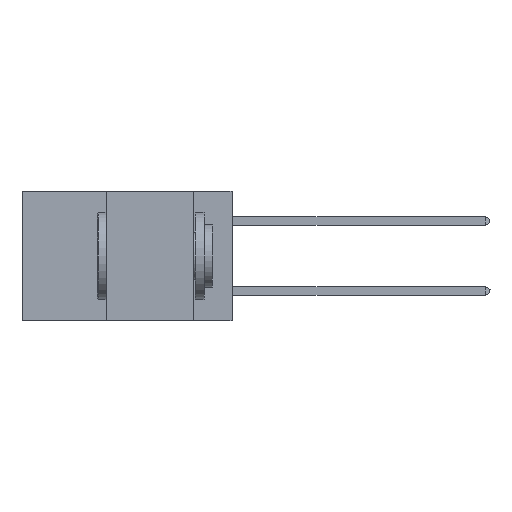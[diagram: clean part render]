
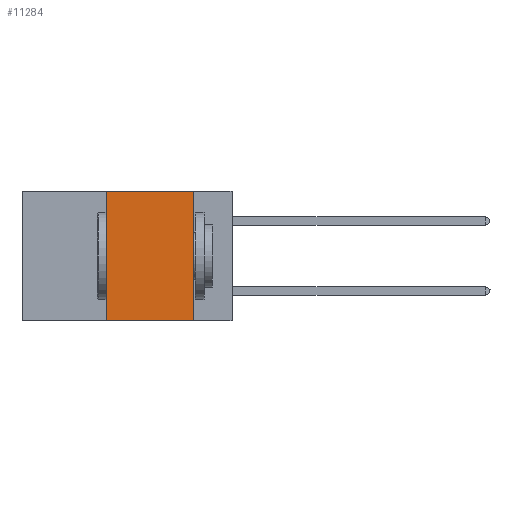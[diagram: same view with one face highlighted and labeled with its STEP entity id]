
A CAD part, left-side view. The second image highlights one B-rep face of the part: STEP entity #11284.
In plain terms, the highlighted planar face has unit normal (-1, 0, 0).
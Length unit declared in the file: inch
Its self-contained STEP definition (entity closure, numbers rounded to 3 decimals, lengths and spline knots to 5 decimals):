
#239 = VERTEX_POINT ( 'NONE', #14572 ) ;
#611 = VERTEX_POINT ( 'NONE', #3948 ) ;
#1262 = VECTOR ( 'NONE', #9452, 39.37008 ) ;
#1735 = CARTESIAN_POINT ( 'NONE',  ( 0., 0.6, 0. ) ) ;
#1811 = DIRECTION ( 'NONE',  ( 0., 0., -1. ) ) ;
#2583 = ORIENTED_EDGE ( 'NONE', *, *, #6250, .F. ) ;
#2960 = VERTEX_POINT ( 'NONE', #4269 ) ;
#3948 = CARTESIAN_POINT ( 'NONE',  ( 0., 0.11, -0.37 ) ) ;
#4269 = CARTESIAN_POINT ( 'NONE',  ( 0., 0.36, 0. ) ) ;
#4355 = CARTESIAN_POINT ( 'NONE',  ( 0., 0.6, -0.37 ) ) ;
#4360 = EDGE_CURVE ( 'NONE', #18378, #2960, #11762, .T. ) ;
#4525 = CARTESIAN_POINT ( 'NONE',  ( 0., 0.36, 0. ) ) ;
#4765 = PLANE ( 'NONE',  #9789 ) ;
#6250 = EDGE_CURVE ( 'NONE', #2960, #239, #18507, .T. ) ;
#6452 = FACE_OUTER_BOUND ( 'NONE', #16123, .T. ) ;
#7163 = ORIENTED_EDGE ( 'NONE', *, *, #9255, .F. ) ;
#7591 = DIRECTION ( 'NONE',  ( 0., 0., -1. ) ) ;
#8311 = VECTOR ( 'NONE', #7591, 39.37008 ) ;
#9255 = EDGE_CURVE ( 'NONE', #239, #611, #13516, .T. ) ;
#9410 = CARTESIAN_POINT ( 'NONE',  ( 0., 0.11, 0. ) ) ;
#9452 = DIRECTION ( 'NONE',  ( 0., 0., 1. ) ) ;
#9789 = AXIS2_PLACEMENT_3D ( 'NONE', #1735, #16121, #1811 ) ;
#10855 = EDGE_CURVE ( 'NONE', #18378, #611, #18445, .T. ) ;
#11206 = VECTOR ( 'NONE', #16896, 39.37008 ) ;
#11284 = ADVANCED_FACE ( 'NONE', ( #6452 ), #4765, .F. ) ;
#11762 = LINE ( 'NONE', #4525, #1262 ) ;
#12622 = ORIENTED_EDGE ( 'NONE', *, *, #10855, .T. ) ;
#13352 = CARTESIAN_POINT ( 'NONE',  ( 0., 0.6, 0. ) ) ;
#13516 = LINE ( 'NONE', #9410, #8311 ) ;
#14572 = CARTESIAN_POINT ( 'NONE',  ( 0., 0.11, 0. ) ) ;
#15679 = CARTESIAN_POINT ( 'NONE',  ( 0., 0.36, -0.37 ) ) ;
#15976 = DIRECTION ( 'NONE',  ( 0., -1., 0. ) ) ;
#16121 = DIRECTION ( 'NONE',  ( 1., 0., 0. ) ) ;
#16123 = EDGE_LOOP ( 'NONE', ( #7163, #2583, #17142, #12622 ) ) ;
#16896 = DIRECTION ( 'NONE',  ( 0., -1., 0. ) ) ;
#17142 = ORIENTED_EDGE ( 'NONE', *, *, #4360, .F. ) ;
#17519 = VECTOR ( 'NONE', #15976, 39.37008 ) ;
#18378 = VERTEX_POINT ( 'NONE', #15679 ) ;
#18445 = LINE ( 'NONE', #4355, #11206 ) ;
#18507 = LINE ( 'NONE', #13352, #17519 ) ;
